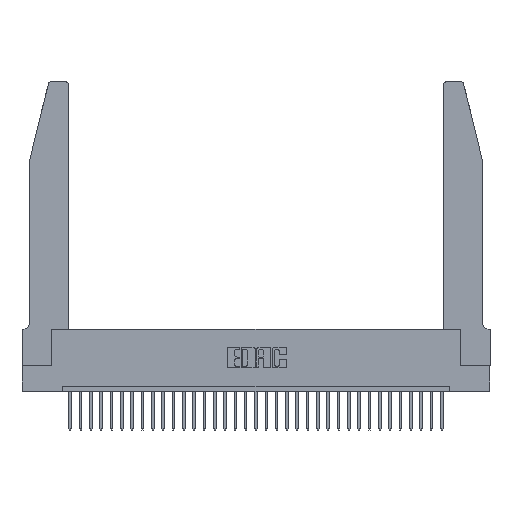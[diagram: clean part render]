
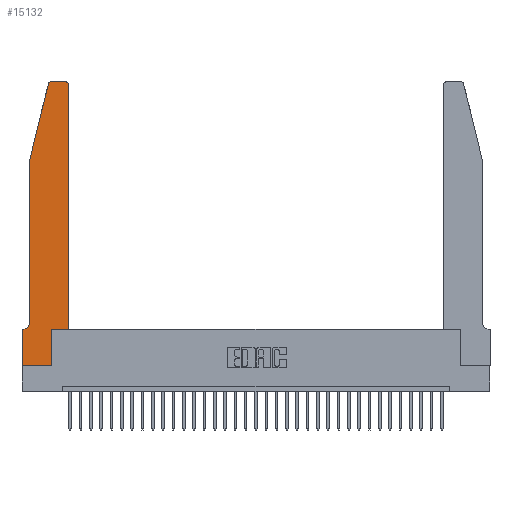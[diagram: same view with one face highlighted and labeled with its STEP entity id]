
A CAD part, top view. The second image highlights one B-rep face of the part: STEP entity #15132.
In plain terms, the highlighted planar face has unit normal (0, 0, 1).
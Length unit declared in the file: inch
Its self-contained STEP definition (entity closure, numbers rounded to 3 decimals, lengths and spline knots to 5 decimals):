
#300 = EDGE_CURVE ( 'NONE', #4166, #5539, #14208, .T. ) ;
#955 = EDGE_CURVE ( 'NONE', #15752, #4424, #27382, .T. ) ;
#1384 = EDGE_CURVE ( 'NONE', #19699, #28518, #24135, .T. ) ;
#1924 = LINE ( 'NONE', #15610, #28413 ) ;
#2151 = ORIENTED_EDGE ( 'NONE', *, *, #5132, .T. ) ;
#2302 = LINE ( 'NONE', #10893, #17969 ) ;
#2618 = VECTOR ( 'NONE', #29691, 39.37008 ) ;
#2716 = ORIENTED_EDGE ( 'NONE', *, *, #955, .T. ) ;
#2915 = DIRECTION ( 'NONE',  ( 1., 0., 0. ) ) ;
#3391 = EDGE_CURVE ( 'NONE', #30493, #13374, #32029, .T. ) ;
#3645 = CARTESIAN_POINT ( 'NONE',  ( 0.2865, 0.35, 0.37 ) ) ;
#4016 = DIRECTION ( 'NONE',  ( 1., 0., 0. ) ) ;
#4166 = VERTEX_POINT ( 'NONE', #25957 ) ;
#4317 = CARTESIAN_POINT ( 'NONE',  ( 0.4505, 0.35, 0.37 ) ) ;
#4424 = VERTEX_POINT ( 'NONE', #12001 ) ;
#4816 = CARTESIAN_POINT ( 'NONE',  ( 0.284, 2.72, 0.37 ) ) ;
#4930 = DIRECTION ( 'NONE',  ( 0., 0., 1. ) ) ;
#5132 = EDGE_CURVE ( 'NONE', #28518, #4166, #13536, .T. ) ;
#5539 = VERTEX_POINT ( 'NONE', #30273 ) ;
#5939 = AXIS2_PLACEMENT_3D ( 'NONE', #17186, #25066, #27417 ) ;
#6383 = CARTESIAN_POINT ( 'NONE',  ( 0., 0., 0.37 ) ) ;
#7063 = PLANE ( 'NONE',  #5939 ) ;
#9009 = CARTESIAN_POINT ( 'NONE',  ( 0., 0., 0.37 ) ) ;
#9265 = VECTOR ( 'NONE', #20117, 39.37008 ) ;
#10051 = ORIENTED_EDGE ( 'NONE', *, *, #28546, .T. ) ;
#10596 = CARTESIAN_POINT ( 'NONE',  ( 0.4505, 0.35, 0.37 ) ) ;
#10703 = DIRECTION ( 'NONE',  ( 0., 1., 0. ) ) ;
#10784 = VECTOR ( 'NONE', #27185, 39.37008 ) ;
#10893 = CARTESIAN_POINT ( 'NONE',  ( 0.2605, 2.75, 0.37 ) ) ;
#11094 = VECTOR ( 'NONE', #18762, 39.37008 ) ;
#11572 = CARTESIAN_POINT ( 'NONE',  ( 0.2865, 0.35, 0.37 ) ) ;
#11585 = CARTESIAN_POINT ( 'NONE',  ( 0., 0., 0.37 ) ) ;
#11943 = LINE ( 'NONE', #26404, #11094 ) ;
#12001 = CARTESIAN_POINT ( 'NONE',  ( 0.4505, 2.72, 0.37 ) ) ;
#12326 = ORIENTED_EDGE ( 'NONE', *, *, #12905, .T. ) ;
#12905 = EDGE_CURVE ( 'NONE', #17117, #30493, #2302, .T. ) ;
#13151 = CARTESIAN_POINT ( 'NONE',  ( 0.2865, 0., 0.37 ) ) ;
#13374 = VERTEX_POINT ( 'NONE', #15886 ) ;
#13536 = CIRCLE ( 'NONE', #25439, 0.07 ) ;
#14208 = LINE ( 'NONE', #19116, #21392 ) ;
#15051 = EDGE_CURVE ( 'NONE', #15056, #30434, #27486, .T. ) ;
#15056 = VERTEX_POINT ( 'NONE', #11585 ) ;
#15132 = ADVANCED_FACE ( 'NONE', ( #15418 ), #7063, .T. ) ;
#15163 = DIRECTION ( 'NONE',  ( 1., 0., 0. ) ) ;
#15418 = FACE_OUTER_BOUND ( 'NONE', #26515, .T. ) ;
#15610 = CARTESIAN_POINT ( 'NONE',  ( 0.4505, 0.35, 0.37 ) ) ;
#15752 = VERTEX_POINT ( 'NONE', #10596 ) ;
#15886 = CARTESIAN_POINT ( 'NONE',  ( 0.25487, 2.72718, 0.37 ) ) ;
#16030 = LINE ( 'NONE', #6383, #10784 ) ;
#16204 = DIRECTION ( 'NONE',  ( -1., 0., 0. ) ) ;
#16358 = ORIENTED_EDGE ( 'NONE', *, *, #15051, .T. ) ;
#17117 = VERTEX_POINT ( 'NONE', #27028 ) ;
#17186 = CARTESIAN_POINT ( 'NONE',  ( 0., 0.35, 0.37 ) ) ;
#17201 = CARTESIAN_POINT ( 'NONE',  ( 0.0755, 2., 0.37 ) ) ;
#17969 = VECTOR ( 'NONE', #16204, 39.37008 ) ;
#18336 = ORIENTED_EDGE ( 'NONE', *, *, #24735, .T. ) ;
#18411 = DIRECTION ( 'NONE',  ( -1., 0., 0. ) ) ;
#18762 = DIRECTION ( 'NONE',  ( -0.239, -0.971, 0. ) ) ;
#19116 = CARTESIAN_POINT ( 'NONE',  ( 0.0755, 0.35, 0.37 ) ) ;
#19699 = VERTEX_POINT ( 'NONE', #17201 ) ;
#19707 = ORIENTED_EDGE ( 'NONE', *, *, #28748, .T. ) ;
#20117 = DIRECTION ( 'NONE',  ( 0., -1., 0. ) ) ;
#21203 = ORIENTED_EDGE ( 'NONE', *, *, #26642, .T. ) ;
#21392 = VECTOR ( 'NONE', #18411, 39.37008 ) ;
#21567 = AXIS2_PLACEMENT_3D ( 'NONE', #4816, #4930, #15163 ) ;
#21792 = CARTESIAN_POINT ( 'NONE',  ( 0.4205, 2.72, 0.37 ) ) ;
#22029 = VERTEX_POINT ( 'NONE', #3645 ) ;
#23347 = ORIENTED_EDGE ( 'NONE', *, *, #1384, .T. ) ;
#23445 = VECTOR ( 'NONE', #27198, 39.37008 ) ;
#24135 = LINE ( 'NONE', #30356, #9265 ) ;
#24735 = EDGE_CURVE ( 'NONE', #4424, #17117, #27461, .T. ) ;
#25066 = DIRECTION ( 'NONE',  ( 0., 0., 1. ) ) ;
#25439 = AXIS2_PLACEMENT_3D ( 'NONE', #31932, #29220, #26271 ) ;
#25957 = CARTESIAN_POINT ( 'NONE',  ( 0.0055, 0.35, 0.37 ) ) ;
#26271 = DIRECTION ( 'NONE',  ( -1., 0., 0. ) ) ;
#26404 = CARTESIAN_POINT ( 'NONE',  ( 0.0755, 2., 0.37 ) ) ;
#26515 = EDGE_LOOP ( 'NONE', ( #12326, #30861, #19707, #23347, #2151, #31512, #21203, #16358, #30188, #10051, #2716, #18336 ) ) ;
#26642 = EDGE_CURVE ( 'NONE', #5539, #15056, #16030, .T. ) ;
#26812 = DIRECTION ( 'NONE',  ( 0., 0., 1. ) ) ;
#27028 = CARTESIAN_POINT ( 'NONE',  ( 0.4205, 2.75, 0.37 ) ) ;
#27185 = DIRECTION ( 'NONE',  ( 0., -1., 0. ) ) ;
#27198 = DIRECTION ( 'NONE',  ( 1., 0., 0. ) ) ;
#27382 = LINE ( 'NONE', #4317, #28552 ) ;
#27417 = DIRECTION ( 'NONE',  ( 1., 0., 0. ) ) ;
#27461 = CIRCLE ( 'NONE', #27474, 0.03 ) ;
#27474 = AXIS2_PLACEMENT_3D ( 'NONE', #21792, #26812, #4016 ) ;
#27486 = LINE ( 'NONE', #9009, #23445 ) ;
#28413 = VECTOR ( 'NONE', #2915, 39.37008 ) ;
#28518 = VERTEX_POINT ( 'NONE', #31039 ) ;
#28546 = EDGE_CURVE ( 'NONE', #22029, #15752, #1924, .T. ) ;
#28552 = VECTOR ( 'NONE', #10703, 39.37008 ) ;
#28748 = EDGE_CURVE ( 'NONE', #13374, #19699, #11943, .T. ) ;
#29220 = DIRECTION ( 'NONE',  ( 0., 0., -1. ) ) ;
#29691 = DIRECTION ( 'NONE',  ( 0., 1., 0. ) ) ;
#30188 = ORIENTED_EDGE ( 'NONE', *, *, #32284, .T. ) ;
#30273 = CARTESIAN_POINT ( 'NONE',  ( 0., 0.35, 0.37 ) ) ;
#30356 = CARTESIAN_POINT ( 'NONE',  ( 0.0755, 2., 0.37 ) ) ;
#30434 = VERTEX_POINT ( 'NONE', #13151 ) ;
#30493 = VERTEX_POINT ( 'NONE', #31493 ) ;
#30861 = ORIENTED_EDGE ( 'NONE', *, *, #3391, .T. ) ;
#31039 = CARTESIAN_POINT ( 'NONE',  ( 0.0755, 0.42, 0.37 ) ) ;
#31493 = CARTESIAN_POINT ( 'NONE',  ( 0.284, 2.75, 0.37 ) ) ;
#31512 = ORIENTED_EDGE ( 'NONE', *, *, #300, .T. ) ;
#31932 = CARTESIAN_POINT ( 'NONE',  ( 0.0055, 0.42, 0.37 ) ) ;
#32029 = CIRCLE ( 'NONE', #21567, 0.03 ) ;
#32284 = EDGE_CURVE ( 'NONE', #30434, #22029, #32456, .T. ) ;
#32456 = LINE ( 'NONE', #11572, #2618 ) ;
